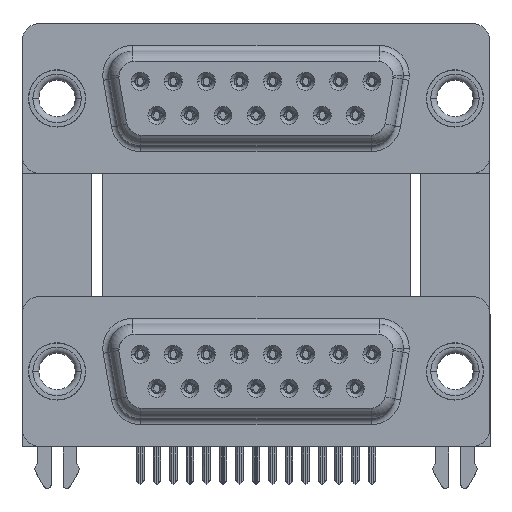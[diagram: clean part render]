
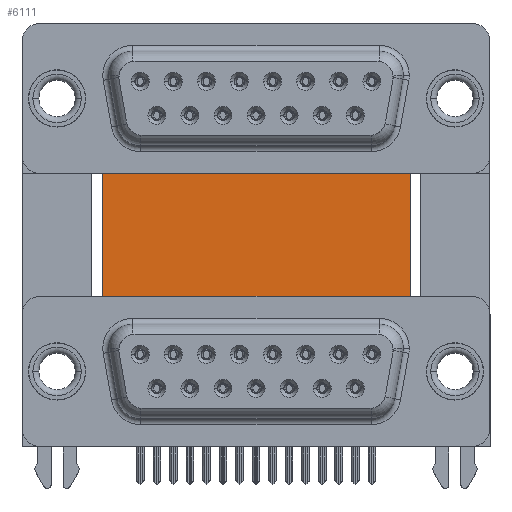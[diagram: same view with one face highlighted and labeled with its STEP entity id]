
A CAD part, top view. The second image highlights one B-rep face of the part: STEP entity #6111.
In plain terms, the highlighted planar face has unit normal (0, 0, 1).
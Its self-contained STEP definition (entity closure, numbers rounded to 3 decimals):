
#2201 = VECTOR ( 'NONE', #48357, 1000. ) ;
#3401 = VERTEX_POINT ( 'NONE', #16285 ) ;
#3699 = EDGE_LOOP ( 'NONE', ( #43962, #5292, #21065, #35484 ) ) ;
#4035 = EDGE_CURVE ( 'NONE', #47619, #3401, #11246, .T. ) ;
#5292 = ORIENTED_EDGE ( 'NONE', *, *, #37455, .F. ) ;
#6111 = ADVANCED_FACE ( 'NONE', ( #41019 ), #7065, .F. ) ;
#7065 = PLANE ( 'NONE',  #31793 ) ;
#9660 = VERTEX_POINT ( 'NONE', #16989 ) ;
#11246 = LINE ( 'NONE', #18182, #17708 ) ;
#13241 = DIRECTION ( 'NONE',  ( 0., -1., 0. ) ) ;
#13736 = CARTESIAN_POINT ( 'NONE',  ( 29.58, 16.585, -12. ) ) ;
#14987 = EDGE_CURVE ( 'NONE', #3401, #42349, #17666, .T. ) ;
#15004 = CARTESIAN_POINT ( 'NONE',  ( 3.79, 16.585, -12. ) ) ;
#16285 = CARTESIAN_POINT ( 'NONE',  ( 3.79, -3.735, -12. ) ) ;
#16989 = CARTESIAN_POINT ( 'NONE',  ( 29.58, 16.585, -12. ) ) ;
#17666 = LINE ( 'NONE', #43705, #25943 ) ;
#17708 = VECTOR ( 'NONE', #18673, 1000. ) ;
#18182 = CARTESIAN_POINT ( 'NONE',  ( 3.79, 16.585, -12. ) ) ;
#18673 = DIRECTION ( 'NONE',  ( 0., -1., 0. ) ) ;
#21065 = ORIENTED_EDGE ( 'NONE', *, *, #32118, .F. ) ;
#21835 = LINE ( 'NONE', #24142, #2201 ) ;
#24142 = CARTESIAN_POINT ( 'NONE',  ( 3.79, 16.585, -12. ) ) ;
#25144 = CARTESIAN_POINT ( 'NONE',  ( 3.79, 16.585, -12. ) ) ;
#25943 = VECTOR ( 'NONE', #40456, 1000. ) ;
#26892 = DIRECTION ( 'NONE',  ( 0., 0., -1. ) ) ;
#30814 = VECTOR ( 'NONE', #13241, 1000. ) ;
#30855 = DIRECTION ( 'NONE',  ( -1., 0., 0. ) ) ;
#31793 = AXIS2_PLACEMENT_3D ( 'NONE', #15004, #26892, #30855 ) ;
#32079 = LINE ( 'NONE', #13736, #30814 ) ;
#32118 = EDGE_CURVE ( 'NONE', #47619, #9660, #21835, .T. ) ;
#35484 = ORIENTED_EDGE ( 'NONE', *, *, #4035, .T. ) ;
#37455 = EDGE_CURVE ( 'NONE', #9660, #42349, #32079, .T. ) ;
#40456 = DIRECTION ( 'NONE',  ( 1., 0., 0. ) ) ;
#41019 = FACE_OUTER_BOUND ( 'NONE', #3699, .T. ) ;
#42349 = VERTEX_POINT ( 'NONE', #46465 ) ;
#43705 = CARTESIAN_POINT ( 'NONE',  ( 3.79, -3.735, -12. ) ) ;
#43962 = ORIENTED_EDGE ( 'NONE', *, *, #14987, .T. ) ;
#46465 = CARTESIAN_POINT ( 'NONE',  ( 29.58, -3.735, -12. ) ) ;
#47619 = VERTEX_POINT ( 'NONE', #25144 ) ;
#48357 = DIRECTION ( 'NONE',  ( 1., 0., 0. ) ) ;
